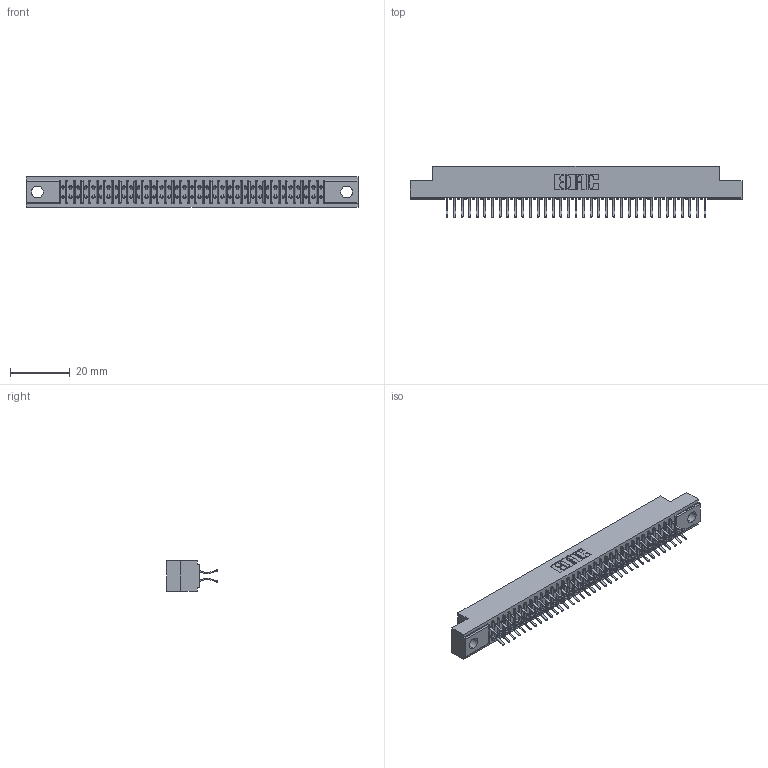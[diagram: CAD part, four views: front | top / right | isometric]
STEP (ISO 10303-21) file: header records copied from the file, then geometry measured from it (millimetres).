
FILE_DESCRIPTION (( 'STEP AP203' ), '1' );
FILE_NAME ('391-070-556-204.STEP', '2018-08-09T14:11:13', ( '' ), ( '' ), 'SwSTEP 2.0', 'SolidWorks 2016', '' );
FILE_SCHEMA (( 'CONFIG_CONTROL_DESIGN' ));
Length unit declared in the file: inch
Products named in the file (3): 341 Part_.156 (3.96) Dia Mounting Holes; 341-292-001_341-292-156; 391-070-556-204
Assembly tree (71 placements, depth 2):
  391-070-556-204
    341 Part_.156 (3.96) Dia Mounting Holes
    341-292-001_341-292-156  x70
Bounding box: 111.12 x 17.07 x 10.16 mm (x, y, z)
Volume: 8116.2 mm3; surface area: 14240 mm2
Topology: 71 solids, 71 shells, 5030 faces, 14597 edges, 9470 vertices
Faces by surface type: plane 2882, cylinder 2008, sphere 72, torus 68
Entity records: 43848 total; most frequent: CARTESIAN_POINT 7295, ORIENTED_EDGE 7246, DIRECTION 7081, EDGE_CURVE 3623, LINE 2921, VECTOR 2921, VERTEX_POINT 2294, AXIS2_PLACEMENT_3D 2080
